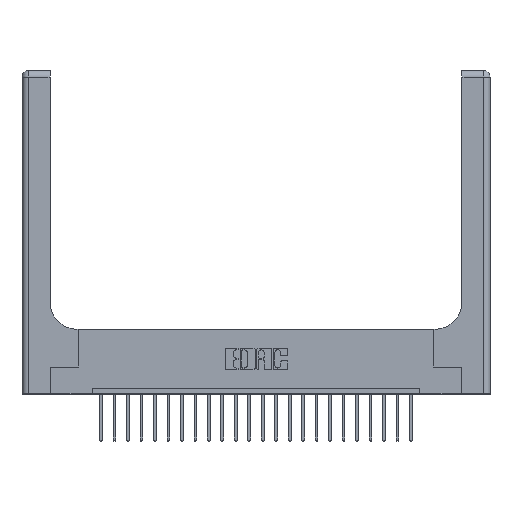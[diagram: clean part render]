
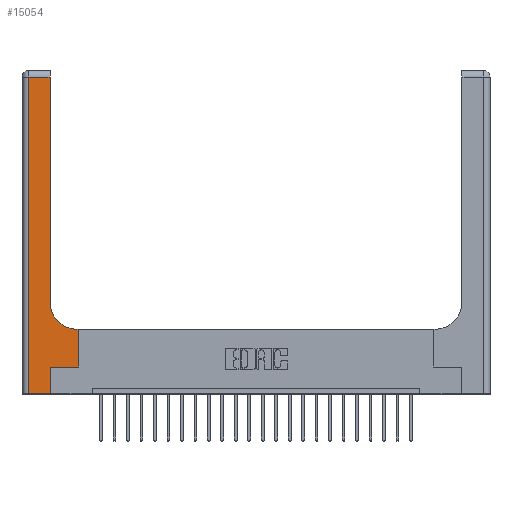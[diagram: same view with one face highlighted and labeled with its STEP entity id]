
A CAD part, top view. The second image highlights one B-rep face of the part: STEP entity #15054.
In plain terms, the highlighted planar face has unit normal (0, 0, 1).
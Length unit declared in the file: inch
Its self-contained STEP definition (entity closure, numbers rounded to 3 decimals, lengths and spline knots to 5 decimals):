
#13 = CARTESIAN_POINT ( 'NONE',  ( 0.265, 0.25, 0.37 ) ) ;
#470 = ORIENTED_EDGE ( 'NONE', *, *, #5859, .T. ) ;
#526 = CIRCLE ( 'NONE', #3070, 0.25 ) ;
#675 = EDGE_CURVE ( 'NONE', #21212, #5896, #4492, .T. ) ;
#677 = ORIENTED_EDGE ( 'NONE', *, *, #2565, .T. ) ;
#935 = AXIS2_PLACEMENT_3D ( 'NONE', #22062, #8189, #1222 ) ;
#1127 = ORIENTED_EDGE ( 'NONE', *, *, #11841, .T. ) ;
#1222 = DIRECTION ( 'NONE',  ( -1., 0., 0. ) ) ;
#1533 = ORIENTED_EDGE ( 'NONE', *, *, #12992, .T. ) ;
#1915 = CARTESIAN_POINT ( 'NONE',  ( 0.26, 3., 0.37 ) ) ;
#2565 = EDGE_CURVE ( 'NONE', #6351, #21212, #3042, .T. ) ;
#2657 = VERTEX_POINT ( 'NONE', #3452 ) ;
#2872 = CARTESIAN_POINT ( 'NONE',  ( 0.06, 0., 0.37 ) ) ;
#3042 = LINE ( 'NONE', #8297, #5782 ) ;
#3070 = AXIS2_PLACEMENT_3D ( 'NONE', #12476, #8787, #5498 ) ;
#3452 = CARTESIAN_POINT ( 'NONE',  ( 0.26, 2.94, 0.37 ) ) ;
#3750 = VECTOR ( 'NONE', #5582, 39.37008 ) ;
#4091 = DIRECTION ( 'NONE',  ( 0., 1., 0. ) ) ;
#4488 = PLANE ( 'NONE',  #935 ) ;
#4492 = LINE ( 'NONE', #14677, #9668 ) ;
#5120 = ORIENTED_EDGE ( 'NONE', *, *, #21107, .T. ) ;
#5498 = DIRECTION ( 'NONE',  ( 1., 0., 0. ) ) ;
#5582 = DIRECTION ( 'NONE',  ( 0., 1., 0. ) ) ;
#5661 = EDGE_CURVE ( 'NONE', #11131, #11617, #14697, .T. ) ;
#5782 = VECTOR ( 'NONE', #10069, 39.37008 ) ;
#5859 = EDGE_CURVE ( 'NONE', #20303, #2657, #19306, .T. ) ;
#5896 = VERTEX_POINT ( 'NONE', #18683 ) ;
#6351 = VERTEX_POINT ( 'NONE', #13 ) ;
#6446 = ORIENTED_EDGE ( 'NONE', *, *, #5661, .T. ) ;
#7363 = VECTOR ( 'NONE', #18517, 39.37008 ) ;
#7400 = ORIENTED_EDGE ( 'NONE', *, *, #675, .T. ) ;
#7768 = ORIENTED_EDGE ( 'NONE', *, *, #11030, .T. ) ;
#8184 = DIRECTION ( 'NONE',  ( 1., 0., 0. ) ) ;
#8189 = DIRECTION ( 'NONE',  ( 0., 0., -1. ) ) ;
#8297 = CARTESIAN_POINT ( 'NONE',  ( 0.265, 0.25, 0.37 ) ) ;
#8787 = DIRECTION ( 'NONE',  ( 0., 0., -1. ) ) ;
#9321 = VECTOR ( 'NONE', #17156, 39.37008 ) ;
#9668 = VECTOR ( 'NONE', #12676, 39.37008 ) ;
#10069 = DIRECTION ( 'NONE',  ( 1., 0., 0. ) ) ;
#10320 = CARTESIAN_POINT ( 'NONE',  ( 0.528, 0.25, 0.37 ) ) ;
#11030 = EDGE_CURVE ( 'NONE', #13439, #6351, #18876, .T. ) ;
#11131 = VERTEX_POINT ( 'NONE', #18417 ) ;
#11617 = VERTEX_POINT ( 'NONE', #2872 ) ;
#11841 = EDGE_CURVE ( 'NONE', #2657, #11131, #18571, .T. ) ;
#11999 = CARTESIAN_POINT ( 'NONE',  ( 0.26, 0.6, 0.37 ) ) ;
#12476 = CARTESIAN_POINT ( 'NONE',  ( 0.51, 0.85, 0.37 ) ) ;
#12676 = DIRECTION ( 'NONE',  ( 0., 1., 0. ) ) ;
#12924 = LINE ( 'NONE', #15168, #21921 ) ;
#12992 = EDGE_CURVE ( 'NONE', #19399, #20303, #526, .T. ) ;
#13439 = VERTEX_POINT ( 'NONE', #17359 ) ;
#14674 = CARTESIAN_POINT ( 'NONE',  ( 0.26, 0.85, 0.37 ) ) ;
#14677 = CARTESIAN_POINT ( 'NONE',  ( 0.528, 0.25, 0.37 ) ) ;
#14697 = LINE ( 'NONE', #21193, #20081 ) ;
#15054 = ADVANCED_FACE ( 'NONE', ( #19760 ), #4488, .F. ) ;
#15168 = CARTESIAN_POINT ( 'NONE',  ( 0., 0., 0.37 ) ) ;
#16967 = EDGE_CURVE ( 'NONE', #5896, #19399, #21587, .T. ) ;
#17156 = DIRECTION ( 'NONE',  ( -1., 0., 0. ) ) ;
#17220 = VECTOR ( 'NONE', #4091, 39.37008 ) ;
#17359 = CARTESIAN_POINT ( 'NONE',  ( 0.265, 0., 0.37 ) ) ;
#18417 = CARTESIAN_POINT ( 'NONE',  ( 0.06, 2.94, 0.37 ) ) ;
#18517 = DIRECTION ( 'NONE',  ( -1., 0., 0. ) ) ;
#18571 = LINE ( 'NONE', #21799, #7363 ) ;
#18683 = CARTESIAN_POINT ( 'NONE',  ( 0.528, 0.6, 0.37 ) ) ;
#18804 = EDGE_LOOP ( 'NONE', ( #470, #1127, #6446, #5120, #7768, #677, #7400, #19957, #1533 ) ) ;
#18876 = LINE ( 'NONE', #21688, #17220 ) ;
#19013 = CARTESIAN_POINT ( 'NONE',  ( 0.51, 0.6, 0.37 ) ) ;
#19306 = LINE ( 'NONE', #1915, #3750 ) ;
#19399 = VERTEX_POINT ( 'NONE', #19013 ) ;
#19760 = FACE_OUTER_BOUND ( 'NONE', #18804, .T. ) ;
#19957 = ORIENTED_EDGE ( 'NONE', *, *, #16967, .T. ) ;
#20081 = VECTOR ( 'NONE', #21639, 39.37008 ) ;
#20303 = VERTEX_POINT ( 'NONE', #14674 ) ;
#21107 = EDGE_CURVE ( 'NONE', #11617, #13439, #12924, .T. ) ;
#21193 = CARTESIAN_POINT ( 'NONE',  ( 0.06, 3., 0.37 ) ) ;
#21212 = VERTEX_POINT ( 'NONE', #10320 ) ;
#21587 = LINE ( 'NONE', #11999, #9321 ) ;
#21639 = DIRECTION ( 'NONE',  ( 0., -1., 0. ) ) ;
#21688 = CARTESIAN_POINT ( 'NONE',  ( 0.265, 0., 0.37 ) ) ;
#21799 = CARTESIAN_POINT ( 'NONE',  ( 0., 2.94, 0.37 ) ) ;
#21921 = VECTOR ( 'NONE', #8184, 39.37008 ) ;
#22062 = CARTESIAN_POINT ( 'NONE',  ( 0., 3., 0.37 ) ) ;
